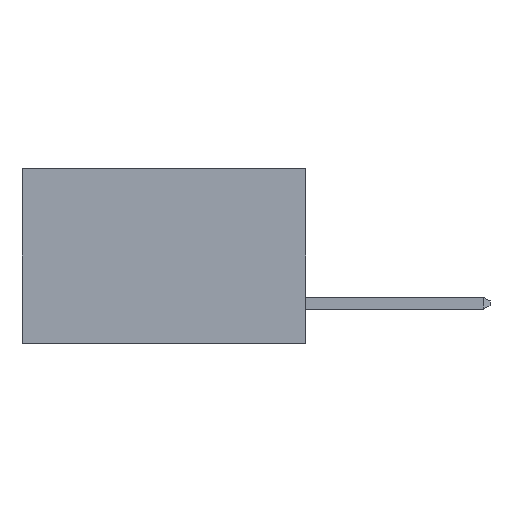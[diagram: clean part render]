
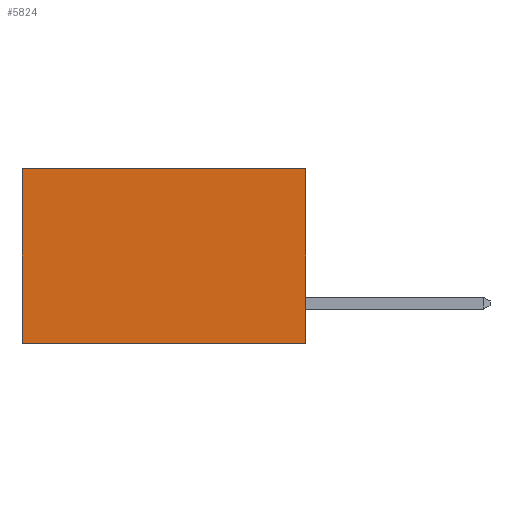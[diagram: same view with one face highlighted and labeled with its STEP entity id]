
A CAD part, left-side view. The second image highlights one B-rep face of the part: STEP entity #5824.
In plain terms, the highlighted planar face has unit normal (-1, 0, 0).
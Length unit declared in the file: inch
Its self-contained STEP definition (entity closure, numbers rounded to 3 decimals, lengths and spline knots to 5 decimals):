
#83 = EDGE_CURVE ( 'NONE', #1973, #8216, #10381, .T. ) ;
#279 = ORIENTED_EDGE ( 'NONE', *, *, #8631, .F. ) ;
#851 = VECTOR ( 'NONE', #6473, 39.37008 ) ;
#1317 = DIRECTION ( 'NONE',  ( 0., 1., 0. ) ) ;
#1973 = VERTEX_POINT ( 'NONE', #8450 ) ;
#2923 = LINE ( 'NONE', #4267, #5716 ) ;
#3098 = CARTESIAN_POINT ( 'NONE',  ( 0.298, 0., 0. ) ) ;
#3406 = EDGE_CURVE ( 'NONE', #10086, #4297, #10598, .T. ) ;
#3796 = AXIS2_PLACEMENT_3D ( 'NONE', #6121, #5297, #8049 ) ;
#3923 = CARTESIAN_POINT ( 'NONE',  ( 0.298, 0.6, 0. ) ) ;
#4223 = CARTESIAN_POINT ( 'NONE',  ( 0.298, 0.6, 0. ) ) ;
#4267 = CARTESIAN_POINT ( 'NONE',  ( 0.298, 0., 0. ) ) ;
#4297 = VERTEX_POINT ( 'NONE', #3923 ) ;
#4747 = CARTESIAN_POINT ( 'NONE',  ( 0.298, 0., 0. ) ) ;
#5297 = DIRECTION ( 'NONE',  ( 1., 0., 0. ) ) ;
#5511 = CARTESIAN_POINT ( 'NONE',  ( 0.298, 0.6, -0.37 ) ) ;
#5716 = VECTOR ( 'NONE', #8755, 39.37008 ) ;
#5824 = ADVANCED_FACE ( 'NONE', ( #6085 ), #6142, .F. ) ;
#6085 = FACE_OUTER_BOUND ( 'NONE', #8630, .T. ) ;
#6121 = CARTESIAN_POINT ( 'NONE',  ( 0.298, 0., 0. ) ) ;
#6142 = PLANE ( 'NONE',  #3796 ) ;
#6473 = DIRECTION ( 'NONE',  ( 0., 1., 0. ) ) ;
#6902 = ORIENTED_EDGE ( 'NONE', *, *, #10925, .T. ) ;
#7878 = VECTOR ( 'NONE', #11456, 39.37008 ) ;
#8049 = DIRECTION ( 'NONE',  ( 0., 0., -1. ) ) ;
#8216 = VERTEX_POINT ( 'NONE', #5511 ) ;
#8221 = VECTOR ( 'NONE', #1317, 39.37008 ) ;
#8450 = CARTESIAN_POINT ( 'NONE',  ( 0.298, 0., -0.37 ) ) ;
#8630 = EDGE_LOOP ( 'NONE', ( #6902, #9865, #279, #10702 ) ) ;
#8631 = EDGE_CURVE ( 'NONE', #10086, #1973, #2923, .T. ) ;
#8755 = DIRECTION ( 'NONE',  ( 0., 0., -1. ) ) ;
#9865 = ORIENTED_EDGE ( 'NONE', *, *, #83, .F. ) ;
#10086 = VERTEX_POINT ( 'NONE', #4747 ) ;
#10266 = LINE ( 'NONE', #4223, #7878 ) ;
#10381 = LINE ( 'NONE', #11089, #851 ) ;
#10598 = LINE ( 'NONE', #3098, #8221 ) ;
#10702 = ORIENTED_EDGE ( 'NONE', *, *, #3406, .T. ) ;
#10925 = EDGE_CURVE ( 'NONE', #4297, #8216, #10266, .T. ) ;
#11089 = CARTESIAN_POINT ( 'NONE',  ( 0.298, 0., -0.37 ) ) ;
#11456 = DIRECTION ( 'NONE',  ( 0., 0., -1. ) ) ;
